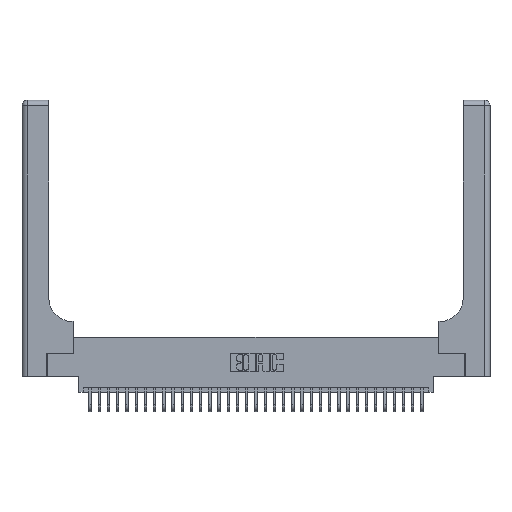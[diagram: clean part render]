
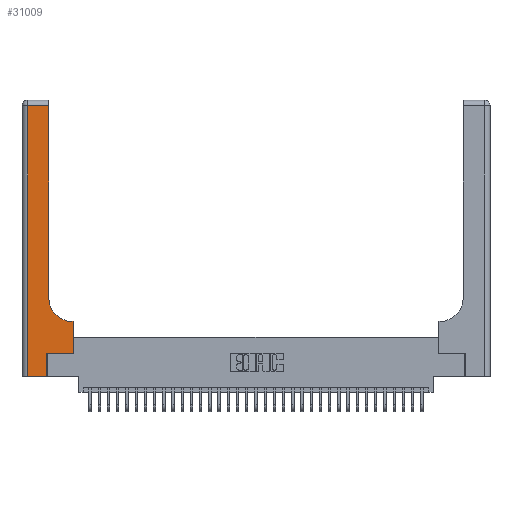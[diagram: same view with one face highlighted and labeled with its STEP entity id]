
A CAD part, top view. The second image highlights one B-rep face of the part: STEP entity #31009.
In plain terms, the highlighted planar face has unit normal (0, 0, 1).
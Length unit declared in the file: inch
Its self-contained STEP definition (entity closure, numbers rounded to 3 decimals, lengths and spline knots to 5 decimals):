
#166 = CARTESIAN_POINT ( 'NONE',  ( 0.2915, 3., 0.37 ) ) ;
#598 = ORIENTED_EDGE ( 'NONE', *, *, #35209, .T. ) ;
#610 = CARTESIAN_POINT ( 'NONE',  ( 0.5415, 0.6, 0.37 ) ) ;
#1346 = DIRECTION ( 'NONE',  ( 0., 0., -1. ) ) ;
#1454 = LINE ( 'NONE', #21267, #6790 ) ;
#1681 = CARTESIAN_POINT ( 'NONE',  ( 0.2915, 0.6, 0.37 ) ) ;
#1778 = CARTESIAN_POINT ( 'NONE',  ( 0., 2.94, 0.37 ) ) ;
#1954 = VECTOR ( 'NONE', #14359, 39.37008 ) ;
#3399 = CIRCLE ( 'NONE', #21133, 0.25 ) ;
#3575 = VERTEX_POINT ( 'NONE', #12883 ) ;
#4370 = DIRECTION ( 'NONE',  ( 1., 0., 0. ) ) ;
#4918 = CARTESIAN_POINT ( 'NONE',  ( 0.5585, 0.25, 0.37 ) ) ;
#5145 = VERTEX_POINT ( 'NONE', #27900 ) ;
#6790 = VECTOR ( 'NONE', #35502, 39.37008 ) ;
#7466 = CARTESIAN_POINT ( 'NONE',  ( 0.5415, 0.85, 0.37 ) ) ;
#8127 = VERTEX_POINT ( 'NONE', #20399 ) ;
#8893 = CARTESIAN_POINT ( 'NONE',  ( 0.5585, 0.25, 0.37 ) ) ;
#9501 = CARTESIAN_POINT ( 'NONE',  ( 0.269, 0.25, 0.37 ) ) ;
#9711 = LINE ( 'NONE', #9501, #31476 ) ;
#10154 = ORIENTED_EDGE ( 'NONE', *, *, #17013, .T. ) ;
#10324 = EDGE_CURVE ( 'NONE', #8127, #23494, #21117, .T. ) ;
#10390 = VECTOR ( 'NONE', #24070, 39.37008 ) ;
#11231 = EDGE_LOOP ( 'NONE', ( #11728, #18269, #10154, #598, #35798, #19176, #16715, #31481, #27050 ) ) ;
#11419 = CARTESIAN_POINT ( 'NONE',  ( 0.06, 2.94, 0.37 ) ) ;
#11728 = ORIENTED_EDGE ( 'NONE', *, *, #31805, .T. ) ;
#11823 = CARTESIAN_POINT ( 'NONE',  ( 0.2915, 0.85, 0.37 ) ) ;
#12437 = DIRECTION ( 'NONE',  ( -1., 0., 0. ) ) ;
#12512 = VERTEX_POINT ( 'NONE', #8893 ) ;
#12883 = CARTESIAN_POINT ( 'NONE',  ( 0.269, 0.25, 0.37 ) ) ;
#13450 = DIRECTION ( 'NONE',  ( 0., 1., 0. ) ) ;
#14359 = DIRECTION ( 'NONE',  ( 0., -1., 0. ) ) ;
#14853 = LINE ( 'NONE', #4918, #25501 ) ;
#14982 = VECTOR ( 'NONE', #28462, 39.37008 ) ;
#16647 = DIRECTION ( 'NONE',  ( -1., 0., 0. ) ) ;
#16715 = ORIENTED_EDGE ( 'NONE', *, *, #26887, .T. ) ;
#17013 = EDGE_CURVE ( 'NONE', #33402, #21852, #22359, .T. ) ;
#17138 = EDGE_CURVE ( 'NONE', #23444, #3575, #1454, .T. ) ;
#18269 = ORIENTED_EDGE ( 'NONE', *, *, #22379, .T. ) ;
#18280 = LINE ( 'NONE', #1778, #10390 ) ;
#19176 = ORIENTED_EDGE ( 'NONE', *, *, #31325, .T. ) ;
#19434 = EDGE_CURVE ( 'NONE', #23494, #25128, #3399, .T. ) ;
#19680 = LINE ( 'NONE', #26471, #30328 ) ;
#20399 = CARTESIAN_POINT ( 'NONE',  ( 0.5585, 0.6, 0.37 ) ) ;
#20483 = CARTESIAN_POINT ( 'NONE',  ( 0.269, 0., 0.37 ) ) ;
#21117 = LINE ( 'NONE', #1681, #33614 ) ;
#21133 = AXIS2_PLACEMENT_3D ( 'NONE', #7466, #1346, #4370 ) ;
#21267 = CARTESIAN_POINT ( 'NONE',  ( 0.269, 0., 0.37 ) ) ;
#21852 = VERTEX_POINT ( 'NONE', #36111 ) ;
#22084 = PLANE ( 'NONE',  #36169 ) ;
#22359 = LINE ( 'NONE', #30994, #1954 ) ;
#22379 = EDGE_CURVE ( 'NONE', #5145, #33402, #18280, .T. ) ;
#22448 = CARTESIAN_POINT ( 'NONE',  ( 0., 3., 0.37 ) ) ;
#22549 = LINE ( 'NONE', #166, #14982 ) ;
#23444 = VERTEX_POINT ( 'NONE', #20483 ) ;
#23494 = VERTEX_POINT ( 'NONE', #610 ) ;
#24070 = DIRECTION ( 'NONE',  ( -1., 0., 0. ) ) ;
#25128 = VERTEX_POINT ( 'NONE', #11823 ) ;
#25501 = VECTOR ( 'NONE', #13450, 39.37008 ) ;
#26342 = DIRECTION ( 'NONE',  ( 1., 0., 0. ) ) ;
#26471 = CARTESIAN_POINT ( 'NONE',  ( 0., 0., 0.37 ) ) ;
#26887 = EDGE_CURVE ( 'NONE', #12512, #8127, #14853, .T. ) ;
#27050 = ORIENTED_EDGE ( 'NONE', *, *, #19434, .T. ) ;
#27783 = DIRECTION ( 'NONE',  ( 0., 0., -1. ) ) ;
#27900 = CARTESIAN_POINT ( 'NONE',  ( 0.2915, 2.94, 0.37 ) ) ;
#28462 = DIRECTION ( 'NONE',  ( 0., 1., 0. ) ) ;
#29341 = DIRECTION ( 'NONE',  ( 1., 0., 0. ) ) ;
#30328 = VECTOR ( 'NONE', #26342, 39.37008 ) ;
#30994 = CARTESIAN_POINT ( 'NONE',  ( 0.06, 3., 0.37 ) ) ;
#31009 = ADVANCED_FACE ( 'NONE', ( #34581 ), #22084, .F. ) ;
#31325 = EDGE_CURVE ( 'NONE', #3575, #12512, #9711, .T. ) ;
#31476 = VECTOR ( 'NONE', #29341, 39.37008 ) ;
#31481 = ORIENTED_EDGE ( 'NONE', *, *, #10324, .T. ) ;
#31805 = EDGE_CURVE ( 'NONE', #25128, #5145, #22549, .T. ) ;
#33402 = VERTEX_POINT ( 'NONE', #11419 ) ;
#33614 = VECTOR ( 'NONE', #12437, 39.37008 ) ;
#34581 = FACE_OUTER_BOUND ( 'NONE', #11231, .T. ) ;
#35209 = EDGE_CURVE ( 'NONE', #21852, #23444, #19680, .T. ) ;
#35502 = DIRECTION ( 'NONE',  ( 0., 1., 0. ) ) ;
#35798 = ORIENTED_EDGE ( 'NONE', *, *, #17138, .T. ) ;
#36111 = CARTESIAN_POINT ( 'NONE',  ( 0.06, 0., 0.37 ) ) ;
#36169 = AXIS2_PLACEMENT_3D ( 'NONE', #22448, #27783, #16647 ) ;
